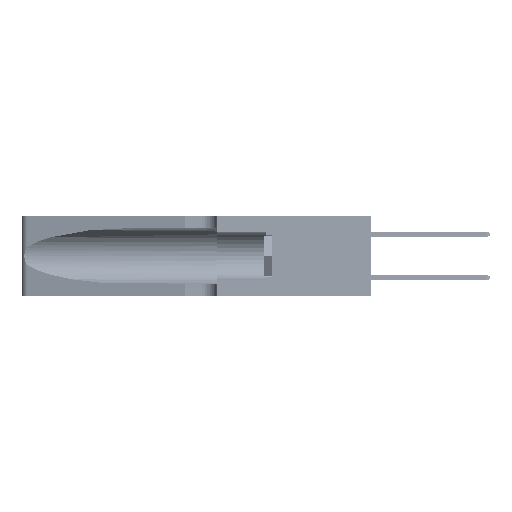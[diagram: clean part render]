
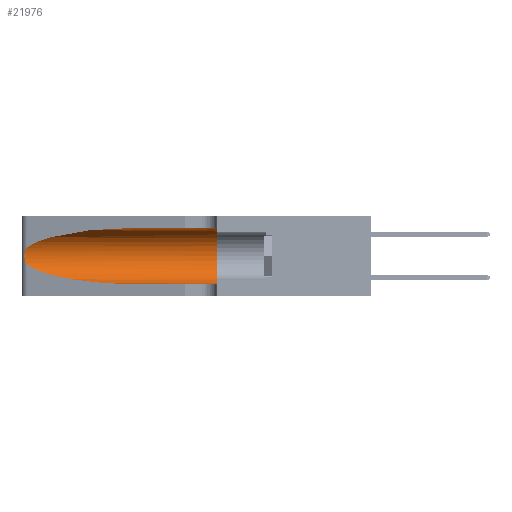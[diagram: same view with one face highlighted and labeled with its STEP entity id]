
A CAD part, left-side view. The second image highlights one B-rep face of the part: STEP entity #21976.
In plain terms, the highlighted cylindrical face has radius 3.308 mm (diameter 6.617 mm), a partial arc.
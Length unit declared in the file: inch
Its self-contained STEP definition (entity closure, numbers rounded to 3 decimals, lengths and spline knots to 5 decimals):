
#1097 = EDGE_CURVE ( 'NONE', #52820, #39502, #37289, .T. ) ;
#1203 = DIRECTION ( 'NONE',  ( 0., 0., 1. ) ) ;
#1537 = CARTESIAN_POINT ( 'NONE',  ( 0.1305, 1.61858, 0.05475 ) ) ;
#3394 = VERTEX_POINT ( 'NONE', #44027 ) ;
#3712 = AXIS2_PLACEMENT_3D ( 'NONE', #51886, #26819, #1203 ) ;
#4927 = CARTESIAN_POINT ( 'NONE',  ( 0.25787, 1.23484, 0.2124 ) ) ;
#5359 = CARTESIAN_POINT ( 'NONE',  ( 0.1305, 0.72297, 0.31525 ) ) ;
#5852 = DIRECTION ( 'NONE',  ( 0., -1., 0. ) ) ;
#6064 = VERTEX_POINT ( 'NONE', #9770 ) ;
#8655 = CARTESIAN_POINT ( 'NONE',  ( 0.25487, 1.22718, 0.14631 ) ) ;
#9258 = CARTESIAN_POINT ( 'NONE',  ( 0.26018, 1.23835, 0.19895 ) ) ;
#9770 = CARTESIAN_POINT ( 'NONE',  ( 0.1305, 0.72297, 0.05475 ) ) ;
#9924 = CYLINDRICAL_SURFACE ( 'NONE', #13139, 0.13025 ) ;
#11330 = VECTOR ( 'NONE', #5852, 39.37008 ) ;
#12365 = CARTESIAN_POINT ( 'NONE',  ( 0.18966, 0.96281, 0.31525 ) ) ;
#12936 = CARTESIAN_POINT ( 'NONE',  ( 0.18966, 0.96281, 0.05475 ) ) ;
#13139 = AXIS2_PLACEMENT_3D ( 'NONE', #43613, #52005, #35209 ) ;
#13533 = CARTESIAN_POINT ( 'NONE',  ( 0.26075, 1.23896, 0.178 ) ) ;
#13832 = VECTOR ( 'NONE', #23344, 39.37008 ) ;
#14948 = ORIENTED_EDGE ( 'NONE', *, *, #32575, .T. ) ;
#15999 = ORIENTED_EDGE ( 'NONE', *, *, #22780, .F. ) ;
#16672 = CARTESIAN_POINT ( 'NONE',  ( 0.1305, 0.72297, 0.31525 ) ) ;
#17288 = ORIENTED_EDGE ( 'NONE', *, *, #1097, .F. ) ;
#17848 = CARTESIAN_POINT ( 'NONE',  ( 0.25856, 1.23593, 0.16098 ) ) ;
#20790 = ORIENTED_EDGE ( 'NONE', *, *, #38156, .T. ) ;
#20892 = CARTESIAN_POINT ( 'NONE',  ( 0.1305, 0.35, 0.31525 ) ) ;
#21032 = VERTEX_POINT ( 'NONE', #5359 ) ;
#21385 = CARTESIAN_POINT ( 'NONE',  ( 0.2373, 1.15595, 0.08982 ) ) ;
#21976 = ADVANCED_FACE ( 'NONE', ( #43671 ), #9924, .F. ) ;
#21984 = CARTESIAN_POINT ( 'NONE',  ( 0.25487, 1.22718, 0.22369 ) ) ;
#22171 = CARTESIAN_POINT ( 'NONE',  ( 0.25639, 1.23186, 0.15144 ) ) ;
#22780 = EDGE_CURVE ( 'NONE', #21032, #52820, #47502, .T. ) ;
#23344 = DIRECTION ( 'NONE',  ( 0., -1., 0. ) ) ;
#23547 = ORIENTED_EDGE ( 'NONE', *, *, #47867, .T. ) ;
#24914 =( BOUNDED_CURVE ( )  B_SPLINE_CURVE ( 3, ( #8655, #21385, #12936, #42525 ),
 .UNSPECIFIED., .F., .F. ) 
 B_SPLINE_CURVE_WITH_KNOTS ( ( 4, 4 ),
 ( 3.44316, 4.71239 ),
 .UNSPECIFIED. ) 
 CURVE ( )  GEOMETRIC_REPRESENTATION_ITEM ( )  RATIONAL_B_SPLINE_CURVE ( ( 1., 0.87, 0.87, 1. ) ) 
 REPRESENTATION_ITEM ( '' )  );
#26430 = CARTESIAN_POINT ( 'NONE',  ( 0.25487, 1.22718, 0.14631 ) ) ;
#26819 = DIRECTION ( 'NONE',  ( 0., 1., 0. ) ) ;
#28664 = EDGE_LOOP ( 'NONE', ( #42280, #23547, #14948, #20790, #17288, #15999 ) ) ;
#28819 = CARTESIAN_POINT ( 'NONE',  ( 0.25487, 1.22718, 0.22369 ) ) ;
#29485 = CARTESIAN_POINT ( 'NONE',  ( 0.25487, 1.22718, 0.22369 ) ) ;
#30473 = CARTESIAN_POINT ( 'NONE',  ( 0.25639, 1.23184, 0.21858 ) ) ;
#30497 = VERTEX_POINT ( 'NONE', #28819 ) ;
#31067 = CARTESIAN_POINT ( 'NONE',  ( 0.1305, 0.35, 0.05475 ) ) ;
#32575 = EDGE_CURVE ( 'NONE', #3394, #6064, #24914, .T. ) ;
#34710 = CARTESIAN_POINT ( 'NONE',  ( 0.25854, 1.2359, 0.20912 ) ) ;
#35209 = DIRECTION ( 'NONE',  ( 0., 0., -1. ) ) ;
#37289 = CIRCLE ( 'NONE', #3712, 0.13025 ) ;
#38156 = EDGE_CURVE ( 'NONE', #6064, #39502, #45075, .T. ) ;
#38912 = CARTESIAN_POINT ( 'NONE',  ( 0.26075, 1.23896, 0.19203 ) ) ;
#39502 = VERTEX_POINT ( 'NONE', #31067 ) ;
#40076 = CARTESIAN_POINT ( 'NONE',  ( 0.1305, 1.61858, 0.31525 ) ) ;
#40380 =( BOUNDED_CURVE ( )  B_SPLINE_CURVE ( 3, ( #16672, #12365, #54543, #29485 ),
 .UNSPECIFIED., .F., .T. ) 
 B_SPLINE_CURVE_WITH_KNOTS ( ( 4, 4 ),
 ( 1.5708, 2.84003 ),
 .UNSPECIFIED. ) 
 CURVE ( )  GEOMETRIC_REPRESENTATION_ITEM ( )  RATIONAL_B_SPLINE_CURVE ( ( 1., 0.87, 0.87, 1. ) ) 
 REPRESENTATION_ITEM ( '' )  );
#42280 = ORIENTED_EDGE ( 'NONE', *, *, #50710, .T. ) ;
#42525 = CARTESIAN_POINT ( 'NONE',  ( 0.1305, 0.72297, 0.05475 ) ) ;
#42916 = CARTESIAN_POINT ( 'NONE',  ( 0.25555, 1.22994, 0.2215 ) ) ;
#43098 = CARTESIAN_POINT ( 'NONE',  ( 0.26017, 1.23833, 0.17102 ) ) ;
#43613 = CARTESIAN_POINT ( 'NONE',  ( 0.1305, 1.61858, 0.185 ) ) ;
#43671 = FACE_OUTER_BOUND ( 'NONE', #28664, .T. ) ;
#44027 = CARTESIAN_POINT ( 'NONE',  ( 0.25487, 1.22718, 0.14631 ) ) ;
#45075 = LINE ( 'NONE', #1537, #11330 ) ;
#47316 = CARTESIAN_POINT ( 'NONE',  ( 0.25789, 1.23486, 0.15765 ) ) ;
#47502 = LINE ( 'NONE', #40076, #13832 ) ;
#47867 = EDGE_CURVE ( 'NONE', #30497, #3394, #50086, .T. ) ;
#50086 = B_SPLINE_CURVE_WITH_KNOTS ( 'NONE', 3,
 ( #21984, #42916, #30473, #4927, #34710, #9258, #38912, #13533, #43098, #17848, #47316, #22171, #51495, #26430 ),
 .UNSPECIFIED., .F., .F.,
 ( 4, 2, 2, 2, 2, 2, 4 ),
 ( 0., 0.00027, 0.00053, 0.00107, 0.0016, 0.00187, 0.00214 ),
 .UNSPECIFIED. ) ;
#50710 = EDGE_CURVE ( 'NONE', #21032, #30497, #40380, .T. ) ;
#51495 = CARTESIAN_POINT ( 'NONE',  ( 0.25555, 1.22993, 0.14849 ) ) ;
#51886 = CARTESIAN_POINT ( 'NONE',  ( 0.1305, 0.35, 0.185 ) ) ;
#52005 = DIRECTION ( 'NONE',  ( 0., -1., 0. ) ) ;
#52820 = VERTEX_POINT ( 'NONE', #20892 ) ;
#54543 = CARTESIAN_POINT ( 'NONE',  ( 0.2373, 1.15595, 0.28018 ) ) ;
